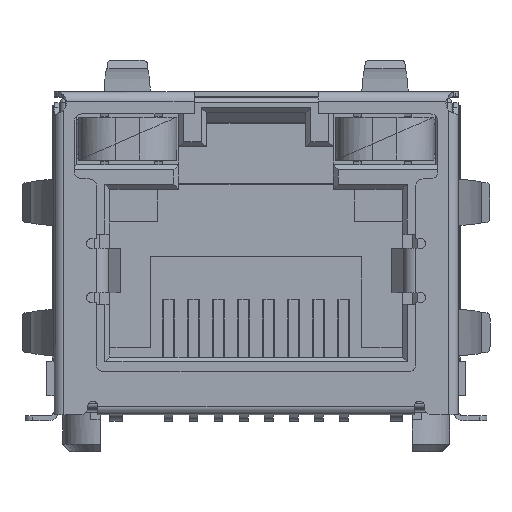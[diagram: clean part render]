
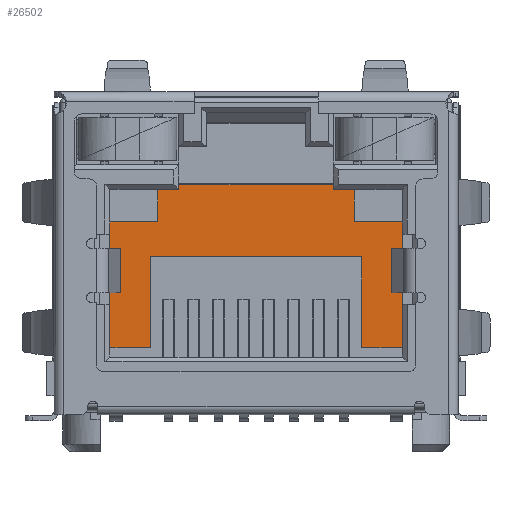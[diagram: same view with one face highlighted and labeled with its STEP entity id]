
A CAD part, top view. The second image highlights one B-rep face of the part: STEP entity #26502.
In plain terms, the highlighted planar face has unit normal (0, 0, 1).
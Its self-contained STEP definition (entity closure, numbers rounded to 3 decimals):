
#73 = CARTESIAN_POINT ( 'NONE',  ( 11.975, 9.08, -12. ) ) ;
#188 = LINE ( 'NONE', #11769, #4793 ) ;
#392 = EDGE_CURVE ( 'NONE', #17278, #26570, #7631, .T. ) ;
#570 = CARTESIAN_POINT ( 'NONE',  ( 12.275, 6.35, -12. ) ) ;
#885 = ORIENTED_EDGE ( 'NONE', *, *, #11577, .T. ) ;
#1091 = DIRECTION ( 'NONE',  ( 0., -1., 0. ) ) ;
#1151 = VERTEX_POINT ( 'NONE', #8893 ) ;
#1298 = ORIENTED_EDGE ( 'NONE', *, *, #4625, .T. ) ;
#1587 = CARTESIAN_POINT ( 'NONE',  ( 4.825, 2.45, -12. ) ) ;
#2112 = EDGE_CURVE ( 'NONE', #8682, #34542, #3419, .T. ) ;
#2731 = EDGE_CURVE ( 'NONE', #11557, #33987, #15410, .T. ) ;
#2934 = CARTESIAN_POINT ( 'NONE',  ( 12.275, 2.45, -12. ) ) ;
#3137 = ORIENTED_EDGE ( 'NONE', *, *, #10418, .T. ) ;
#3419 = LINE ( 'NONE', #1587, #12143 ) ;
#3542 = ORIENTED_EDGE ( 'NONE', *, *, #24395, .T. ) ;
#4625 = EDGE_CURVE ( 'NONE', #14946, #1151, #25993, .T. ) ;
#4793 = VECTOR ( 'NONE', #1091, 1000. ) ;
#4925 = DIRECTION ( 'NONE',  ( -1., 0., 0. ) ) ;
#5499 = DIRECTION ( 'NONE',  ( -1., 0., 0. ) ) ;
#5881 = EDGE_CURVE ( 'NONE', #33987, #31582, #17583, .T. ) ;
#6496 = EDGE_CURVE ( 'NONE', #11922, #27618, #27549, .T. ) ;
#7631 = LINE ( 'NONE', #33290, #23471 ) ;
#7684 = VECTOR ( 'NONE', #5499, 1000. ) ;
#8210 = VECTOR ( 'NONE', #22005, 1000. ) ;
#8238 = ORIENTED_EDGE ( 'NONE', *, *, #12976, .F. ) ;
#8682 = VERTEX_POINT ( 'NONE', #11887 ) ;
#8893 = CARTESIAN_POINT ( 'NONE',  ( 11.975, 7.78, -12. ) ) ;
#8955 = CARTESIAN_POINT ( 'NONE',  ( 2.02, 2.65, -12. ) ) ;
#9077 = CARTESIAN_POINT ( 'NONE',  ( 13.93, 7.78, -12. ) ) ;
#9306 = CARTESIAN_POINT ( 'NONE',  ( 11.125, 9.28, -12. ) ) ;
#9438 = DIRECTION ( 'NONE',  ( -1., 0., 0. ) ) ;
#9439 = CARTESIAN_POINT ( 'NONE',  ( 3.675, 6.35, -12. ) ) ;
#9586 = ORIENTED_EDGE ( 'NONE', *, *, #33105, .F. ) ;
#9794 = CARTESIAN_POINT ( 'NONE',  ( 2.02, 2.25, -12. ) ) ;
#10418 = EDGE_CURVE ( 'NONE', #33507, #8682, #31112, .T. ) ;
#11433 = LINE ( 'NONE', #17851, #29319 ) ;
#11557 = VERTEX_POINT ( 'NONE', #17242 ) ;
#11577 = EDGE_CURVE ( 'NONE', #20215, #21844, #34384, .T. ) ;
#11769 = CARTESIAN_POINT ( 'NONE',  ( 13.93, 9.08, -12. ) ) ;
#11787 = DIRECTION ( 'NONE',  ( 0., -1., 0. ) ) ;
#11887 = CARTESIAN_POINT ( 'NONE',  ( 4.825, 9.28, -12. ) ) ;
#11922 = VERTEX_POINT ( 'NONE', #570 ) ;
#11980 = ORIENTED_EDGE ( 'NONE', *, *, #2112, .T. ) ;
#11989 = CARTESIAN_POINT ( 'NONE',  ( 11.975, 7.78, -12. ) ) ;
#12143 = VECTOR ( 'NONE', #11787, 1000. ) ;
#12417 = DIRECTION ( 'NONE',  ( 1., 0., 0. ) ) ;
#12449 = DIRECTION ( 'NONE',  ( 1., 0., 0. ) ) ;
#12600 = DIRECTION ( 'NONE',  ( 0., 1., 0. ) ) ;
#12653 = LINE ( 'NONE', #17114, #13485 ) ;
#12976 = EDGE_CURVE ( 'NONE', #11557, #21844, #31318, .T. ) ;
#13168 = CARTESIAN_POINT ( 'NONE',  ( 3.675, 2.45, -12. ) ) ;
#13440 = VECTOR ( 'NONE', #12600, 1000. ) ;
#13485 = VECTOR ( 'NONE', #24791, 1000. ) ;
#13771 = CARTESIAN_POINT ( 'NONE',  ( 13.93, 2.65, -12. ) ) ;
#13989 = CARTESIAN_POINT ( 'NONE',  ( 4.825, 9.08, -12. ) ) ;
#14069 = LINE ( 'NONE', #21555, #8210 ) ;
#14179 = VERTEX_POINT ( 'NONE', #14976 ) ;
#14336 = EDGE_LOOP ( 'NONE', ( #885, #8238, #31958, #33378, #29337, #21007, #20954, #9586, #1298, #21337, #27878, #18172, #3137, #11980, #33153, #3542 ) ) ;
#14626 = AXIS2_PLACEMENT_3D ( 'NONE', #15082, #31124, #12417 ) ;
#14649 = LINE ( 'NONE', #11989, #29224 ) ;
#14946 = VERTEX_POINT ( 'NONE', #9077 ) ;
#14976 = CARTESIAN_POINT ( 'NONE',  ( 3.975, 9.08, -12. ) ) ;
#15082 = CARTESIAN_POINT ( 'NONE',  ( 2.02, 2.45, -12. ) ) ;
#15410 = LINE ( 'NONE', #8955, #17940 ) ;
#15450 = VECTOR ( 'NONE', #32608, 1000. ) ;
#15498 = VECTOR ( 'NONE', #26413, 1000. ) ;
#15939 = VECTOR ( 'NONE', #21094, 1000. ) ;
#17114 = CARTESIAN_POINT ( 'NONE',  ( 13.93, 2.65, -12. ) ) ;
#17242 = CARTESIAN_POINT ( 'NONE',  ( 2.02, 2.65, -12. ) ) ;
#17278 = VERTEX_POINT ( 'NONE', #73 ) ;
#17583 = LINE ( 'NONE', #13168, #15498 ) ;
#17851 = CARTESIAN_POINT ( 'NONE',  ( 2.02, 9.08, -12. ) ) ;
#17879 = LINE ( 'NONE', #29163, #24922 ) ;
#17940 = VECTOR ( 'NONE', #12449, 1000. ) ;
#18006 = CARTESIAN_POINT ( 'NONE',  ( 4.825, 9.28, -12. ) ) ;
#18172 = ORIENTED_EDGE ( 'NONE', *, *, #25755, .T. ) ;
#18252 = EDGE_CURVE ( 'NONE', #31582, #11922, #14069, .T. ) ;
#18686 = CARTESIAN_POINT ( 'NONE',  ( 3.975, 7.78, -12. ) ) ;
#18959 = VECTOR ( 'NONE', #19817, 1000. ) ;
#19429 = CARTESIAN_POINT ( 'NONE',  ( 2.02, 7.78, -12. ) ) ;
#19817 = DIRECTION ( 'NONE',  ( -1., 0., 0. ) ) ;
#20215 = VERTEX_POINT ( 'NONE', #18686 ) ;
#20239 = CARTESIAN_POINT ( 'NONE',  ( 3.675, 2.65, -12. ) ) ;
#20475 = EDGE_CURVE ( 'NONE', #34542, #14179, #11433, .T. ) ;
#20954 = ORIENTED_EDGE ( 'NONE', *, *, #33370, .F. ) ;
#21007 = ORIENTED_EDGE ( 'NONE', *, *, #6496, .T. ) ;
#21094 = DIRECTION ( 'NONE',  ( 0., -1., 0. ) ) ;
#21203 = CARTESIAN_POINT ( 'NONE',  ( 2.02, 7.78, -12. ) ) ;
#21337 = ORIENTED_EDGE ( 'NONE', *, *, #24149, .T. ) ;
#21555 = CARTESIAN_POINT ( 'NONE',  ( 2.02, 6.35, -12. ) ) ;
#21844 = VERTEX_POINT ( 'NONE', #19429 ) ;
#22005 = DIRECTION ( 'NONE',  ( 1., 0., 0. ) ) ;
#22401 = FACE_OUTER_BOUND ( 'NONE', #14336, .T. ) ;
#22485 = DIRECTION ( 'NONE',  ( 0., 1., 0. ) ) ;
#23471 = VECTOR ( 'NONE', #9438, 1000. ) ;
#24070 = CARTESIAN_POINT ( 'NONE',  ( 12.275, 2.65, -12. ) ) ;
#24149 = EDGE_CURVE ( 'NONE', #1151, #17278, #14649, .T. ) ;
#24395 = EDGE_CURVE ( 'NONE', #14179, #20215, #30425, .T. ) ;
#24585 = CARTESIAN_POINT ( 'NONE',  ( 3.975, 9.08, -12. ) ) ;
#24791 = DIRECTION ( 'NONE',  ( -1., 0., 0. ) ) ;
#24922 = VECTOR ( 'NONE', #34326, 1000. ) ;
#25755 = EDGE_CURVE ( 'NONE', #26570, #33507, #17879, .T. ) ;
#25788 = DIRECTION ( 'NONE',  ( -1., 0., 0. ) ) ;
#25993 = LINE ( 'NONE', #21203, #7684 ) ;
#26413 = DIRECTION ( 'NONE',  ( 0., 1., 0. ) ) ;
#26502 = ADVANCED_FACE ( 'NONE', ( #22401 ), #28295, .T. ) ;
#26570 = VERTEX_POINT ( 'NONE', #26678 ) ;
#26678 = CARTESIAN_POINT ( 'NONE',  ( 11.125, 9.08, -12. ) ) ;
#27549 = LINE ( 'NONE', #2934, #15939 ) ;
#27618 = VERTEX_POINT ( 'NONE', #24070 ) ;
#27878 = ORIENTED_EDGE ( 'NONE', *, *, #392, .T. ) ;
#28295 = PLANE ( 'NONE',  #14626 ) ;
#28526 = VERTEX_POINT ( 'NONE', #13771 ) ;
#29163 = CARTESIAN_POINT ( 'NONE',  ( 11.125, 2.45, -12. ) ) ;
#29224 = VECTOR ( 'NONE', #22485, 1000. ) ;
#29319 = VECTOR ( 'NONE', #4925, 1000. ) ;
#29337 = ORIENTED_EDGE ( 'NONE', *, *, #18252, .T. ) ;
#30425 = LINE ( 'NONE', #24585, #15450 ) ;
#31112 = LINE ( 'NONE', #18006, #31925 ) ;
#31124 = DIRECTION ( 'NONE',  ( 0., 0., 1. ) ) ;
#31318 = LINE ( 'NONE', #9794, #13440 ) ;
#31582 = VERTEX_POINT ( 'NONE', #9439 ) ;
#31925 = VECTOR ( 'NONE', #25788, 1000. ) ;
#31958 = ORIENTED_EDGE ( 'NONE', *, *, #2731, .T. ) ;
#32608 = DIRECTION ( 'NONE',  ( 0., -1., 0. ) ) ;
#33105 = EDGE_CURVE ( 'NONE', #14946, #28526, #188, .T. ) ;
#33153 = ORIENTED_EDGE ( 'NONE', *, *, #20475, .T. ) ;
#33185 = CARTESIAN_POINT ( 'NONE',  ( 2.02, 7.78, -12. ) ) ;
#33290 = CARTESIAN_POINT ( 'NONE',  ( 2.02, 9.08, -12. ) ) ;
#33370 = EDGE_CURVE ( 'NONE', #28526, #27618, #12653, .T. ) ;
#33378 = ORIENTED_EDGE ( 'NONE', *, *, #5881, .T. ) ;
#33507 = VERTEX_POINT ( 'NONE', #9306 ) ;
#33987 = VERTEX_POINT ( 'NONE', #20239 ) ;
#34326 = DIRECTION ( 'NONE',  ( 0., 1., 0. ) ) ;
#34384 = LINE ( 'NONE', #33185, #18959 ) ;
#34542 = VERTEX_POINT ( 'NONE', #13989 ) ;
